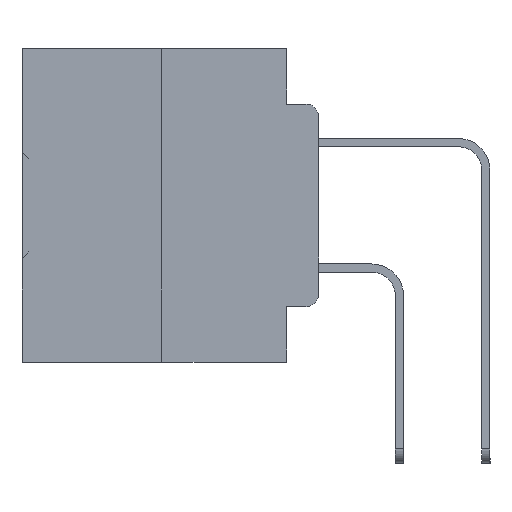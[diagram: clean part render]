
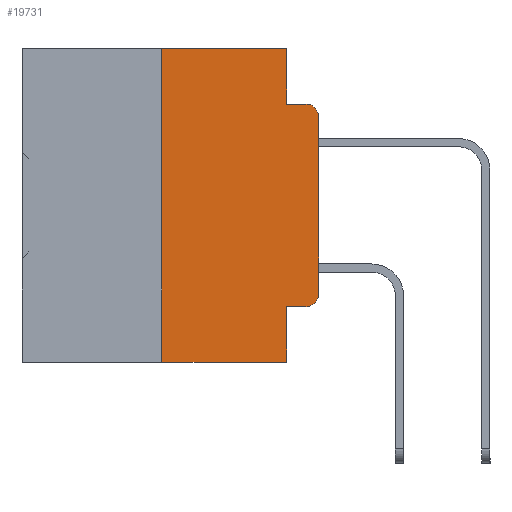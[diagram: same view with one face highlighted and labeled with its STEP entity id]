
A CAD part, left-side view. The second image highlights one B-rep face of the part: STEP entity #19731.
In plain terms, the highlighted planar face has unit normal (-1, 0, 0).
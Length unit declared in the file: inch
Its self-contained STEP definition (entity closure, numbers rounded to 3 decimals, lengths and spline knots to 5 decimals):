
#1109 = CARTESIAN_POINT ( 'NONE',  ( 0., 0.051, 0. ) ) ;
#1519 = EDGE_CURVE ( 'NONE', #8150, #27232, #12736, .T. ) ;
#2636 = CARTESIAN_POINT ( 'NONE',  ( 0., 0.051, -0.4115 ) ) ;
#2649 = VERTEX_POINT ( 'NONE', #25090 ) ;
#2724 = ORIENTED_EDGE ( 'NONE', *, *, #18115, .F. ) ;
#2805 = VECTOR ( 'NONE', #20259, 39.37008 ) ;
#2966 = EDGE_CURVE ( 'NONE', #37293, #2649, #30115, .T. ) ;
#3158 = DIRECTION ( 'NONE',  ( 0., -1., 0. ) ) ;
#4288 = EDGE_CURVE ( 'NONE', #31196, #39592, #21439, .T. ) ;
#5289 = AXIS2_PLACEMENT_3D ( 'NONE', #39621, #30586, #12197 ) ;
#5768 = CARTESIAN_POINT ( 'NONE',  ( 0., 0.051, 0. ) ) ;
#6194 = ORIENTED_EDGE ( 'NONE', *, *, #2966, .T. ) ;
#7525 = CARTESIAN_POINT ( 'NONE',  ( 0., 0.051, -0.4115 ) ) ;
#7649 = LINE ( 'NONE', #7784, #31279 ) ;
#7784 = CARTESIAN_POINT ( 'NONE',  ( 0., 0.473, -0.5 ) ) ;
#7905 = DIRECTION ( 'NONE',  ( -1., 0., 0. ) ) ;
#8150 = VERTEX_POINT ( 'NONE', #35406 ) ;
#8677 = DIRECTION ( 'NONE',  ( -1., 0., 0. ) ) ;
#8767 = EDGE_CURVE ( 'NONE', #38949, #34288, #7649, .T. ) ;
#9601 = AXIS2_PLACEMENT_3D ( 'NONE', #36381, #8677, #16689 ) ;
#10407 = VERTEX_POINT ( 'NONE', #33932 ) ;
#11452 = FACE_OUTER_BOUND ( 'NONE', #32471, .T. ) ;
#12197 = DIRECTION ( 'NONE',  ( 0., 0., -1. ) ) ;
#12736 = CIRCLE ( 'NONE', #9601, 0.02 ) ;
#14615 = EDGE_CURVE ( 'NONE', #25530, #8150, #35156, .T. ) ;
#15924 = LINE ( 'NONE', #16625, #31284 ) ;
#16397 = ORIENTED_EDGE ( 'NONE', *, *, #23308, .T. ) ;
#16625 = CARTESIAN_POINT ( 'NONE',  ( 0., 0.051, 0. ) ) ;
#16689 = DIRECTION ( 'NONE',  ( 0., 0., -1. ) ) ;
#16865 = CARTESIAN_POINT ( 'NONE',  ( 0., 0.25, -0.5 ) ) ;
#17201 = CARTESIAN_POINT ( 'NONE',  ( 0., 0.25, 0. ) ) ;
#17730 = EDGE_CURVE ( 'NONE', #37293, #34288, #38449, .T. ) ;
#17789 = ORIENTED_EDGE ( 'NONE', *, *, #14615, .T. ) ;
#18115 = EDGE_CURVE ( 'NONE', #39592, #10407, #15924, .T. ) ;
#18428 = CARTESIAN_POINT ( 'NONE',  ( 0., 0.051, -0.5 ) ) ;
#18687 = DIRECTION ( 'NONE',  ( 0., -1., 0. ) ) ;
#18848 = VECTOR ( 'NONE', #35997, 39.37008 ) ;
#19242 = ORIENTED_EDGE ( 'NONE', *, *, #4288, .F. ) ;
#19695 = ORIENTED_EDGE ( 'NONE', *, *, #1519, .T. ) ;
#19731 = ADVANCED_FACE ( 'NONE', ( #11452 ), #27512, .F. ) ;
#20259 = DIRECTION ( 'NONE',  ( 0., 0., 1. ) ) ;
#20877 = CARTESIAN_POINT ( 'NONE',  ( 0., 0.051, -0.0885 ) ) ;
#21439 = LINE ( 'NONE', #27812, #36752 ) ;
#21690 = ORIENTED_EDGE ( 'NONE', *, *, #17730, .F. ) ;
#21703 = AXIS2_PLACEMENT_3D ( 'NONE', #26380, #7905, #29439 ) ;
#22005 = LINE ( 'NONE', #20877, #29164 ) ;
#22152 = ORIENTED_EDGE ( 'NONE', *, *, #32819, .F. ) ;
#23303 = DIRECTION ( 'NONE',  ( 0., -1., 0. ) ) ;
#23308 = EDGE_CURVE ( 'NONE', #2649, #25530, #23721, .T. ) ;
#23650 = CARTESIAN_POINT ( 'NONE',  ( 0., 0.25, 0. ) ) ;
#23721 = CIRCLE ( 'NONE', #21703, 0.02 ) ;
#23970 = DIRECTION ( 'NONE',  ( 0., -1., 0. ) ) ;
#25090 = CARTESIAN_POINT ( 'NONE',  ( 0., 0.02, -0.4115 ) ) ;
#25530 = VERTEX_POINT ( 'NONE', #26444 ) ;
#25888 = DIRECTION ( 'NONE',  ( 0., 0., -1. ) ) ;
#26380 = CARTESIAN_POINT ( 'NONE',  ( 0., 0.02, -0.3915 ) ) ;
#26444 = CARTESIAN_POINT ( 'NONE',  ( 0., 0., -0.3915 ) ) ;
#27232 = VERTEX_POINT ( 'NONE', #29555 ) ;
#27497 = LINE ( 'NONE', #17201, #2805 ) ;
#27512 = PLANE ( 'NONE',  #5289 ) ;
#27812 = CARTESIAN_POINT ( 'NONE',  ( 0., 0.473, 0. ) ) ;
#28422 = VECTOR ( 'NONE', #25888, 39.37008 ) ;
#29164 = VECTOR ( 'NONE', #23970, 39.37008 ) ;
#29439 = DIRECTION ( 'NONE',  ( 0., 0., -1. ) ) ;
#29555 = CARTESIAN_POINT ( 'NONE',  ( 0., 0.02, -0.0885 ) ) ;
#30115 = LINE ( 'NONE', #2636, #36327 ) ;
#30586 = DIRECTION ( 'NONE',  ( 1., 0., 0. ) ) ;
#30608 = EDGE_CURVE ( 'NONE', #10407, #27232, #22005, .T. ) ;
#31196 = VERTEX_POINT ( 'NONE', #23650 ) ;
#31279 = VECTOR ( 'NONE', #23303, 39.37008 ) ;
#31284 = VECTOR ( 'NONE', #38039, 39.37008 ) ;
#32471 = EDGE_LOOP ( 'NONE', ( #17789, #19695, #37911, #2724, #19242, #22152, #33181, #21690, #6194, #16397 ) ) ;
#32819 = EDGE_CURVE ( 'NONE', #38949, #31196, #27497, .T. ) ;
#32927 = CARTESIAN_POINT ( 'NONE',  ( 0., 0., 0. ) ) ;
#33181 = ORIENTED_EDGE ( 'NONE', *, *, #8767, .T. ) ;
#33932 = CARTESIAN_POINT ( 'NONE',  ( 0., 0.051, -0.0885 ) ) ;
#34288 = VERTEX_POINT ( 'NONE', #18428 ) ;
#35156 = LINE ( 'NONE', #32927, #18848 ) ;
#35406 = CARTESIAN_POINT ( 'NONE',  ( 0., 0., -0.1085 ) ) ;
#35997 = DIRECTION ( 'NONE',  ( 0., 0., 1. ) ) ;
#36327 = VECTOR ( 'NONE', #3158, 39.37008 ) ;
#36381 = CARTESIAN_POINT ( 'NONE',  ( 0., 0.02, -0.1085 ) ) ;
#36752 = VECTOR ( 'NONE', #18687, 39.37008 ) ;
#37293 = VERTEX_POINT ( 'NONE', #7525 ) ;
#37911 = ORIENTED_EDGE ( 'NONE', *, *, #30608, .F. ) ;
#38039 = DIRECTION ( 'NONE',  ( 0., 0., -1. ) ) ;
#38449 = LINE ( 'NONE', #1109, #28422 ) ;
#38949 = VERTEX_POINT ( 'NONE', #16865 ) ;
#39592 = VERTEX_POINT ( 'NONE', #5768 ) ;
#39621 = CARTESIAN_POINT ( 'NONE',  ( 0., 0.473, 0. ) ) ;
